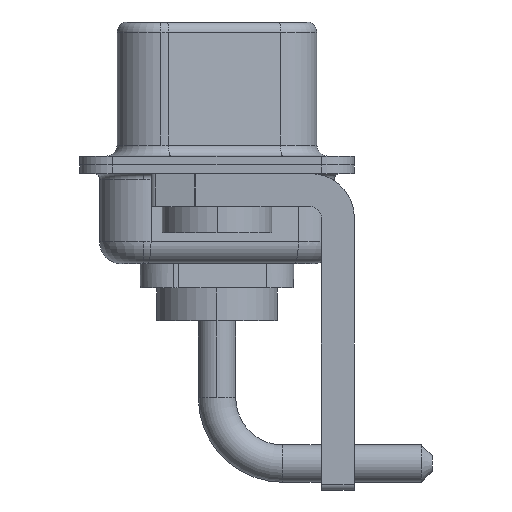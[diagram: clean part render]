
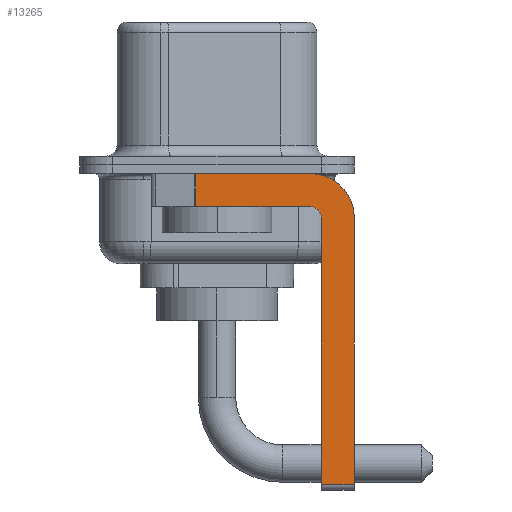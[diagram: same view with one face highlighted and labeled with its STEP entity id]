
A CAD part, left-side view. The second image highlights one B-rep face of the part: STEP entity #13265.
In plain terms, the highlighted planar face has unit normal (-1, 0, 0).
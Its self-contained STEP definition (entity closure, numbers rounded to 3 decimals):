
#488 = ORIENTED_EDGE ( 'NONE', *, *, #9278, .F. ) ;
#1237 = DIRECTION ( 'NONE',  ( 0., -1., 0. ) ) ;
#1327 = CARTESIAN_POINT ( 'NONE',  ( -2.9, -6.25, -2.4 ) ) ;
#1385 = ORIENTED_EDGE ( 'NONE', *, *, #15125, .T. ) ;
#1753 = VERTEX_POINT ( 'NONE', #2423 ) ;
#1800 = CARTESIAN_POINT ( 'NONE',  ( -2.9, 0.978, -1.9 ) ) ;
#1846 = CARTESIAN_POINT ( 'NONE',  ( -2.9, -4.75, -2.4 ) ) ;
#2082 = VECTOR ( 'NONE', #6467, 1000. ) ;
#2181 = EDGE_CURVE ( 'NONE', #3366, #7201, #6068, .T. ) ;
#2423 = CARTESIAN_POINT ( 'NONE',  ( -2.9, -4.25, -1.9 ) ) ;
#2542 = AXIS2_PLACEMENT_3D ( 'NONE', #3518, #9491, #5839 ) ;
#2632 = ORIENTED_EDGE ( 'NONE', *, *, #5313, .F. ) ;
#2896 = LINE ( 'NONE', #7625, #2082 ) ;
#3107 = CARTESIAN_POINT ( 'NONE',  ( -2.9, 0.978, -1.9 ) ) ;
#3281 = FACE_OUTER_BOUND ( 'NONE', #12854, .T. ) ;
#3366 = VERTEX_POINT ( 'NONE', #4024 ) ;
#3518 = CARTESIAN_POINT ( 'NONE',  ( -2.9, -4.25, -2.4 ) ) ;
#4024 = CARTESIAN_POINT ( 'NONE',  ( -2.9, -6.25, -2.4 ) ) ;
#4068 = EDGE_CURVE ( 'NONE', #6282, #3366, #12896, .T. ) ;
#4748 = CARTESIAN_POINT ( 'NONE',  ( -2.9, -4.25, -14.55 ) ) ;
#4881 = ORIENTED_EDGE ( 'NONE', *, *, #14412, .F. ) ;
#5013 = DIRECTION ( 'NONE',  ( 0., -1., 0. ) ) ;
#5090 = CARTESIAN_POINT ( 'NONE',  ( -2.9, 3., -0.4 ) ) ;
#5313 = EDGE_CURVE ( 'NONE', #1753, #14443, #2896, .T. ) ;
#5327 = DIRECTION ( 'NONE',  ( -1., 0., 0. ) ) ;
#5357 = ORIENTED_EDGE ( 'NONE', *, *, #10351, .F. ) ;
#5467 = DIRECTION ( 'NONE',  ( 0., 0., 1. ) ) ;
#5807 = VERTEX_POINT ( 'NONE', #13210 ) ;
#5839 = DIRECTION ( 'NONE',  ( 0., 0., -1. ) ) ;
#5852 = VECTOR ( 'NONE', #11708, 1000. ) ;
#6068 = LINE ( 'NONE', #1327, #5852 ) ;
#6282 = VERTEX_POINT ( 'NONE', #12102 ) ;
#6467 = DIRECTION ( 'NONE',  ( 0., 1., 0. ) ) ;
#6720 = AXIS2_PLACEMENT_3D ( 'NONE', #9101, #5327, #5467 ) ;
#6728 = CARTESIAN_POINT ( 'NONE',  ( -2.9, -6.25, -14.55 ) ) ;
#6911 = CARTESIAN_POINT ( 'NONE',  ( -2.9, -4.25, -2.4 ) ) ;
#6973 = ORIENTED_EDGE ( 'NONE', *, *, #4068, .F. ) ;
#7201 = VERTEX_POINT ( 'NONE', #6728 ) ;
#7226 = LINE ( 'NONE', #4748, #10265 ) ;
#7625 = CARTESIAN_POINT ( 'NONE',  ( -2.9, -4.25, -1.9 ) ) ;
#7933 = VECTOR ( 'NONE', #13943, 1000. ) ;
#8083 = PLANE ( 'NONE',  #2542 ) ;
#8212 = AXIS2_PLACEMENT_3D ( 'NONE', #6911, #12951, #14969 ) ;
#9057 = ORIENTED_EDGE ( 'NONE', *, *, #9427, .T. ) ;
#9101 = CARTESIAN_POINT ( 'NONE',  ( -2.9, -4.25, -2.4 ) ) ;
#9278 = EDGE_CURVE ( 'NONE', #12151, #11283, #9861, .T. ) ;
#9427 = EDGE_CURVE ( 'NONE', #5807, #14443, #14874, .T. ) ;
#9491 = DIRECTION ( 'NONE',  ( 1., 0., 0. ) ) ;
#9861 = LINE ( 'NONE', #14655, #11138 ) ;
#10265 = VECTOR ( 'NONE', #1237, 1000. ) ;
#10351 = EDGE_CURVE ( 'NONE', #11283, #1753, #11923, .T. ) ;
#10880 = LINE ( 'NONE', #5090, #12969 ) ;
#11138 = VECTOR ( 'NONE', #12407, 1000. ) ;
#11283 = VERTEX_POINT ( 'NONE', #1846 ) ;
#11708 = DIRECTION ( 'NONE',  ( 0., 0., -1. ) ) ;
#11923 = CIRCLE ( 'NONE', #6720, 0.5 ) ;
#12051 = CARTESIAN_POINT ( 'NONE',  ( -2.9, -4.75, -14.55 ) ) ;
#12102 = CARTESIAN_POINT ( 'NONE',  ( -2.9, -4.25, -0.4 ) ) ;
#12151 = VERTEX_POINT ( 'NONE', #12051 ) ;
#12407 = DIRECTION ( 'NONE',  ( 0., 0., 1. ) ) ;
#12854 = EDGE_LOOP ( 'NONE', ( #4881, #9057, #2632, #5357, #488, #1385, #13397, #6973 ) ) ;
#12896 = CIRCLE ( 'NONE', #8212, 2. ) ;
#12951 = DIRECTION ( 'NONE',  ( 1., 0., 0. ) ) ;
#12969 = VECTOR ( 'NONE', #5013, 1000. ) ;
#13210 = CARTESIAN_POINT ( 'NONE',  ( -2.9, 0.978, -0.4 ) ) ;
#13265 = ADVANCED_FACE ( 'NONE', ( #3281 ), #8083, .F. ) ;
#13397 = ORIENTED_EDGE ( 'NONE', *, *, #2181, .F. ) ;
#13943 = DIRECTION ( 'NONE',  ( 0., 0., -1. ) ) ;
#14412 = EDGE_CURVE ( 'NONE', #5807, #6282, #10880, .T. ) ;
#14443 = VERTEX_POINT ( 'NONE', #1800 ) ;
#14655 = CARTESIAN_POINT ( 'NONE',  ( -2.9, -4.75, -14.8 ) ) ;
#14874 = LINE ( 'NONE', #3107, #7933 ) ;
#14969 = DIRECTION ( 'NONE',  ( 0., 0., -1. ) ) ;
#15125 = EDGE_CURVE ( 'NONE', #12151, #7201, #7226, .T. ) ;
